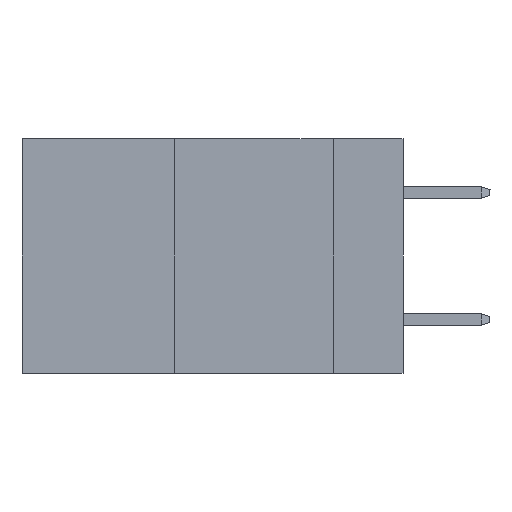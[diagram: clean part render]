
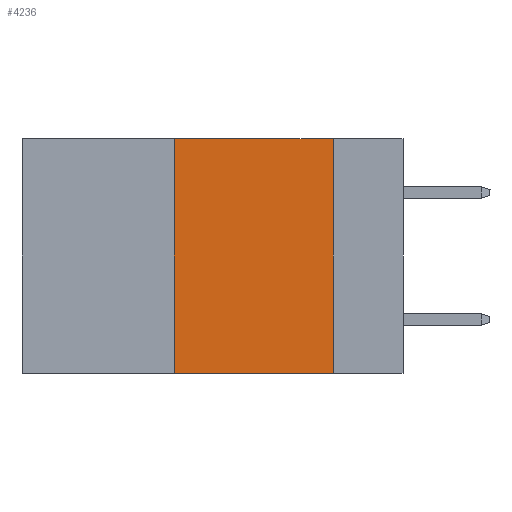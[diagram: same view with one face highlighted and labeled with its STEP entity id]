
A CAD part, left-side view. The second image highlights one B-rep face of the part: STEP entity #4236.
In plain terms, the highlighted planar face has unit normal (-1, 0, 0).
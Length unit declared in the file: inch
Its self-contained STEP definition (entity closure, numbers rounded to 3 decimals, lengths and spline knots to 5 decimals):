
#309 = DIRECTION ( 'NONE',  ( 0., -1., 0. ) ) ;
#315 = VERTEX_POINT ( 'NONE', #3492 ) ;
#417 = DIRECTION ( 'NONE',  ( 0., 0., -1. ) ) ;
#923 = ORIENTED_EDGE ( 'NONE', *, *, #4301, .F. ) ;
#1134 = ORIENTED_EDGE ( 'NONE', *, *, #17806, .T. ) ;
#1629 = VERTEX_POINT ( 'NONE', #20968 ) ;
#2201 = PLANE ( 'NONE',  #20343 ) ;
#3492 = CARTESIAN_POINT ( 'NONE',  ( 0., 0.36, 0. ) ) ;
#3890 = VECTOR ( 'NONE', #14518, 39.37008 ) ;
#4094 = FACE_OUTER_BOUND ( 'NONE', #5718, .T. ) ;
#4236 = ADVANCED_FACE ( 'NONE', ( #4094 ), #2201, .F. ) ;
#4301 = EDGE_CURVE ( 'NONE', #315, #1629, #21017, .T. ) ;
#4832 = LINE ( 'NONE', #8475, #9206 ) ;
#5551 = CARTESIAN_POINT ( 'NONE',  ( 0., 0.36, -0.37 ) ) ;
#5718 = EDGE_LOOP ( 'NONE', ( #21273, #923, #12027, #1134 ) ) ;
#6037 = EDGE_CURVE ( 'NONE', #6706, #315, #7947, .T. ) ;
#6706 = VERTEX_POINT ( 'NONE', #5551 ) ;
#7947 = LINE ( 'NONE', #16204, #3890 ) ;
#8475 = CARTESIAN_POINT ( 'NONE',  ( 0., 0.11, 0. ) ) ;
#9206 = VECTOR ( 'NONE', #21780, 39.37008 ) ;
#10634 = DIRECTION ( 'NONE',  ( 1., 0., 0. ) ) ;
#11058 = CARTESIAN_POINT ( 'NONE',  ( 0., 0.11, -0.37 ) ) ;
#12027 = ORIENTED_EDGE ( 'NONE', *, *, #6037, .F. ) ;
#12474 = VERTEX_POINT ( 'NONE', #11058 ) ;
#12566 = EDGE_CURVE ( 'NONE', #1629, #12474, #4832, .T. ) ;
#12655 = CARTESIAN_POINT ( 'NONE',  ( 0., 0.6, -0.37 ) ) ;
#14518 = DIRECTION ( 'NONE',  ( 0., 0., 1. ) ) ;
#15536 = CARTESIAN_POINT ( 'NONE',  ( 0., 0.6, 0. ) ) ;
#16204 = CARTESIAN_POINT ( 'NONE',  ( 0., 0.36, 0. ) ) ;
#16791 = VECTOR ( 'NONE', #309, 39.37008 ) ;
#17806 = EDGE_CURVE ( 'NONE', #6706, #12474, #21148, .T. ) ;
#19797 = DIRECTION ( 'NONE',  ( 0., -1., 0. ) ) ;
#20343 = AXIS2_PLACEMENT_3D ( 'NONE', #20911, #10634, #417 ) ;
#20911 = CARTESIAN_POINT ( 'NONE',  ( 0., 0.6, 0. ) ) ;
#20968 = CARTESIAN_POINT ( 'NONE',  ( 0., 0.11, 0. ) ) ;
#21017 = LINE ( 'NONE', #15536, #16791 ) ;
#21148 = LINE ( 'NONE', #12655, #21831 ) ;
#21273 = ORIENTED_EDGE ( 'NONE', *, *, #12566, .F. ) ;
#21780 = DIRECTION ( 'NONE',  ( 0., 0., -1. ) ) ;
#21831 = VECTOR ( 'NONE', #19797, 39.37008 ) ;
